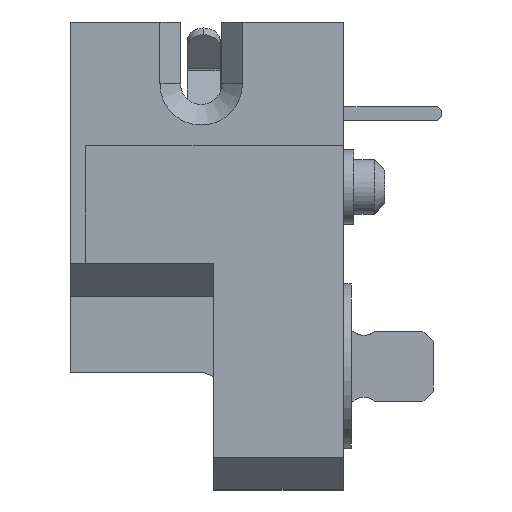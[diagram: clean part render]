
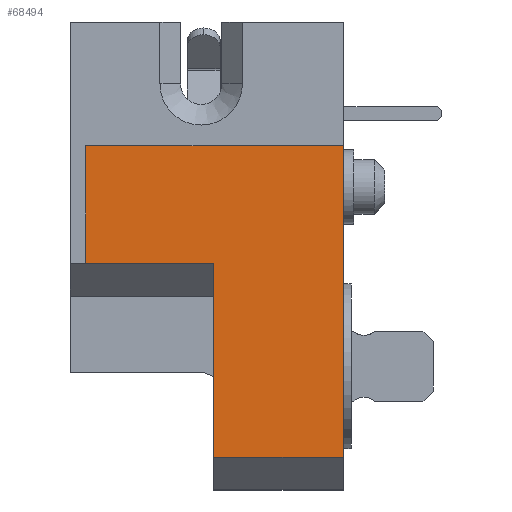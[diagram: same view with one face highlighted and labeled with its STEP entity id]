
A CAD part, left-side view. The second image highlights one B-rep face of the part: STEP entity #68494.
In plain terms, the highlighted planar face has unit normal (-1, 0, 0).
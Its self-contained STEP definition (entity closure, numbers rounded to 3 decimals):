
#5797 = CARTESIAN_POINT ( 'NONE',  ( -26.5, 0., -7.5 ) ) ;
#9788 = VERTEX_POINT ( 'NONE', #53361 ) ;
#9835 = FACE_OUTER_BOUND ( 'NONE', #36443, .T. ) ;
#10700 = CARTESIAN_POINT ( 'NONE',  ( -26.5, 4.89, -2.8 ) ) ;
#10879 = VECTOR ( 'NONE', #60293, 1000. ) ;
#11004 = VECTOR ( 'NONE', #34413, 1000. ) ;
#14302 = DIRECTION ( 'NONE',  ( 0., 0., 1. ) ) ;
#15077 = VERTEX_POINT ( 'NONE', #43917 ) ;
#15472 = EDGE_CURVE ( 'NONE', #9788, #50548, #53982, .T. ) ;
#15566 = CARTESIAN_POINT ( 'NONE',  ( -26.5, 3.125, -7.5 ) ) ;
#16380 = EDGE_CURVE ( 'NONE', #27135, #15077, #27096, .T. ) ;
#17233 = CARTESIAN_POINT ( 'NONE',  ( -26.5, 6.25, 0.05 ) ) ;
#17798 = VERTEX_POINT ( 'NONE', #59136 ) ;
#18191 = LINE ( 'NONE', #49687, #62668 ) ;
#18612 = ORIENTED_EDGE ( 'NONE', *, *, #15472, .F. ) ;
#18664 = LINE ( 'NONE', #67775, #50019 ) ;
#24714 = VERTEX_POINT ( 'NONE', #28726 ) ;
#24945 = LINE ( 'NONE', #28649, #11004 ) ;
#26325 = EDGE_CURVE ( 'NONE', #27135, #24714, #18191, .T. ) ;
#27096 = LINE ( 'NONE', #15566, #10879 ) ;
#27135 = VERTEX_POINT ( 'NONE', #5797 ) ;
#28649 = CARTESIAN_POINT ( 'NONE',  ( -26.5, 3.125, 0.05 ) ) ;
#28726 = CARTESIAN_POINT ( 'NONE',  ( -26.5, 0., 0.05 ) ) ;
#32887 = DIRECTION ( 'NONE',  ( 0., 0., -1. ) ) ;
#33102 = AXIS2_PLACEMENT_3D ( 'NONE', #48771, #43002, #32887 ) ;
#34413 = DIRECTION ( 'NONE',  ( 0., -1., 0. ) ) ;
#36443 = EDGE_LOOP ( 'NONE', ( #65569, #18612, #60184, #46191, #60170, #69685 ) ) ;
#37277 = EDGE_CURVE ( 'NONE', #50548, #24714, #24945, .T. ) ;
#41694 = CARTESIAN_POINT ( 'NONE',  ( -26.5, 6.25, -1.375 ) ) ;
#43002 = DIRECTION ( 'NONE',  ( 1., 0., 0. ) ) ;
#43414 = VECTOR ( 'NONE', #53285, 1000. ) ;
#43753 = EDGE_CURVE ( 'NONE', #15077, #17798, #18664, .T. ) ;
#43917 = CARTESIAN_POINT ( 'NONE',  ( -26.5, 3.15, -7.5 ) ) ;
#46191 = ORIENTED_EDGE ( 'NONE', *, *, #43753, .F. ) ;
#47489 = LINE ( 'NONE', #10700, #43414 ) ;
#48771 = CARTESIAN_POINT ( 'NONE',  ( -26.5, 3.125, -3.725 ) ) ;
#49687 = CARTESIAN_POINT ( 'NONE',  ( -26.5, 0., -2.625 ) ) ;
#50019 = VECTOR ( 'NONE', #63409, 1000. ) ;
#50548 = VERTEX_POINT ( 'NONE', #17233 ) ;
#53285 = DIRECTION ( 'NONE',  ( 0., -1., 0. ) ) ;
#53361 = CARTESIAN_POINT ( 'NONE',  ( -26.5, 6.25, -2.8 ) ) ;
#53982 = LINE ( 'NONE', #41694, #59200 ) ;
#54776 = DIRECTION ( 'NONE',  ( 0., 0., 1. ) ) ;
#55250 = PLANE ( 'NONE',  #33102 ) ;
#59136 = CARTESIAN_POINT ( 'NONE',  ( -26.5, 3.15, -2.8 ) ) ;
#59200 = VECTOR ( 'NONE', #14302, 1000. ) ;
#60170 = ORIENTED_EDGE ( 'NONE', *, *, #16380, .F. ) ;
#60184 = ORIENTED_EDGE ( 'NONE', *, *, #68070, .T. ) ;
#60293 = DIRECTION ( 'NONE',  ( 0., 1., 0. ) ) ;
#62668 = VECTOR ( 'NONE', #54776, 1000. ) ;
#63409 = DIRECTION ( 'NONE',  ( 0., 0., 1. ) ) ;
#65569 = ORIENTED_EDGE ( 'NONE', *, *, #37277, .F. ) ;
#67775 = CARTESIAN_POINT ( 'NONE',  ( -26.5, 3.15, -5.55 ) ) ;
#68070 = EDGE_CURVE ( 'NONE', #9788, #17798, #47489, .T. ) ;
#68494 = ADVANCED_FACE ( 'NONE', ( #9835 ), #55250, .F. ) ;
#69685 = ORIENTED_EDGE ( 'NONE', *, *, #26325, .T. ) ;
